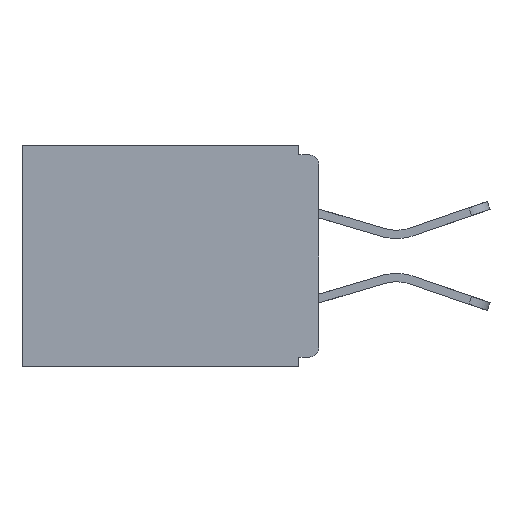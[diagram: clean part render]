
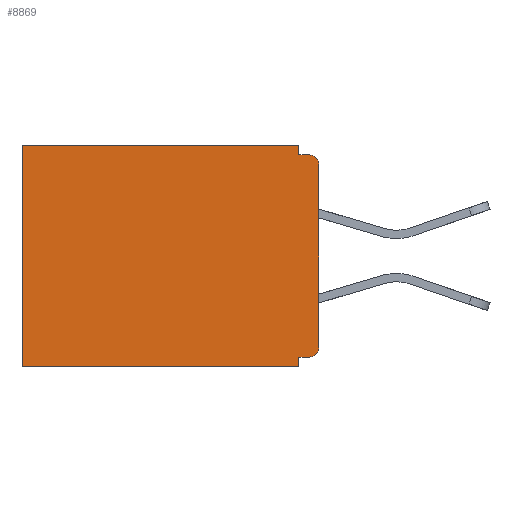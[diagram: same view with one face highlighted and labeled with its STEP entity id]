
A CAD part, left-side view. The second image highlights one B-rep face of the part: STEP entity #8869.
In plain terms, the highlighted planar face has unit normal (-1, 0, 0).
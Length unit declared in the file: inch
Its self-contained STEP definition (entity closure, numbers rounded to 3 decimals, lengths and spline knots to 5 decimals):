
#92 = CIRCLE ( 'NONE', #14591, 0.015 ) ;
#360 = VERTEX_POINT ( 'NONE', #4422 ) ;
#743 = CARTESIAN_POINT ( 'NONE',  ( 0.298, 0.031, -0.343 ) ) ;
#793 = EDGE_CURVE ( 'NONE', #5922, #4514, #23040, .T. ) ;
#941 = ORIENTED_EDGE ( 'NONE', *, *, #23031, .T. ) ;
#2200 = DIRECTION ( 'NONE',  ( -1., 0., 0. ) ) ;
#2765 = DIRECTION ( 'NONE',  ( 0., 0., -1. ) ) ;
#3049 = ORIENTED_EDGE ( 'NONE', *, *, #24527, .F. ) ;
#3358 = EDGE_CURVE ( 'NONE', #14089, #6622, #10035, .T. ) ;
#3411 = CARTESIAN_POINT ( 'NONE',  ( 0.298, 0.46, 0. ) ) ;
#3434 = VECTOR ( 'NONE', #22749, 39.37008 ) ;
#3955 = CARTESIAN_POINT ( 'NONE',  ( 0.298, 0., -0.313 ) ) ;
#4016 = LINE ( 'NONE', #23531, #30515 ) ;
#4174 = DIRECTION ( 'NONE',  ( 1., 0., 0. ) ) ;
#4422 = CARTESIAN_POINT ( 'NONE',  ( 0.298, 0., -0.03 ) ) ;
#4514 = VERTEX_POINT ( 'NONE', #7853 ) ;
#4957 = LINE ( 'NONE', #10898, #3434 ) ;
#5069 = CARTESIAN_POINT ( 'NONE',  ( 0.298, 0.031, -0.343 ) ) ;
#5861 = VECTOR ( 'NONE', #14106, 39.37008 ) ;
#5922 = VERTEX_POINT ( 'NONE', #30896 ) ;
#6333 = ORIENTED_EDGE ( 'NONE', *, *, #13022, .T. ) ;
#6356 = DIRECTION ( 'NONE',  ( -1., 0., 0. ) ) ;
#6622 = VERTEX_POINT ( 'NONE', #3955 ) ;
#7427 = AXIS2_PLACEMENT_3D ( 'NONE', #21047, #4174, #18617 ) ;
#7533 = AXIS2_PLACEMENT_3D ( 'NONE', #28672, #2200, #31295 ) ;
#7853 = CARTESIAN_POINT ( 'NONE',  ( 0.298, 0.015, -0.015 ) ) ;
#7964 = VERTEX_POINT ( 'NONE', #17951 ) ;
#8869 = ADVANCED_FACE ( 'NONE', ( #13870 ), #11394, .F. ) ;
#8871 = ORIENTED_EDGE ( 'NONE', *, *, #20277, .F. ) ;
#10035 = CIRCLE ( 'NONE', #7533, 0.015 ) ;
#10355 = VERTEX_POINT ( 'NONE', #5069 ) ;
#10571 = LINE ( 'NONE', #17393, #11701 ) ;
#10898 = CARTESIAN_POINT ( 'NONE',  ( 0.298, 0., 0. ) ) ;
#11087 = CARTESIAN_POINT ( 'NONE',  ( 0.298, 0., 0. ) ) ;
#11394 = PLANE ( 'NONE',  #7427 ) ;
#11514 = ORIENTED_EDGE ( 'NONE', *, *, #22446, .F. ) ;
#11548 = CARTESIAN_POINT ( 'NONE',  ( 0.298, 0.015, -0.328 ) ) ;
#11701 = VECTOR ( 'NONE', #15026, 39.37008 ) ;
#12139 = VERTEX_POINT ( 'NONE', #27029 ) ;
#12432 = CARTESIAN_POINT ( 'NONE',  ( 0.298, 0.46, 0. ) ) ;
#12556 = EDGE_CURVE ( 'NONE', #30121, #12139, #12691, .T. ) ;
#12691 = LINE ( 'NONE', #12432, #15337 ) ;
#13022 = EDGE_CURVE ( 'NONE', #360, #4514, #92, .T. ) ;
#13870 = FACE_OUTER_BOUND ( 'NONE', #28330, .T. ) ;
#14089 = VERTEX_POINT ( 'NONE', #11548 ) ;
#14106 = DIRECTION ( 'NONE',  ( 0., 0., -1. ) ) ;
#14257 = ORIENTED_EDGE ( 'NONE', *, *, #3358, .T. ) ;
#14581 = ORIENTED_EDGE ( 'NONE', *, *, #793, .F. ) ;
#14591 = AXIS2_PLACEMENT_3D ( 'NONE', #18575, #6356, #28054 ) ;
#15026 = DIRECTION ( 'NONE',  ( 0., 1., 0. ) ) ;
#15048 = DIRECTION ( 'NONE',  ( 0., -1., 0. ) ) ;
#15337 = VECTOR ( 'NONE', #2765, 39.37008 ) ;
#15776 = ORIENTED_EDGE ( 'NONE', *, *, #12556, .T. ) ;
#15803 = ORIENTED_EDGE ( 'NONE', *, *, #16716, .F. ) ;
#16130 = LINE ( 'NONE', #11087, #5861 ) ;
#16716 = EDGE_CURVE ( 'NONE', #14089, #24022, #10571, .T. ) ;
#17195 = CARTESIAN_POINT ( 'NONE',  ( 0.298, 0.031, -0.343 ) ) ;
#17393 = CARTESIAN_POINT ( 'NONE',  ( 0.298, 0., -0.328 ) ) ;
#17511 = CARTESIAN_POINT ( 'NONE',  ( 0.298, 0., -0.015 ) ) ;
#17951 = CARTESIAN_POINT ( 'NONE',  ( 0.298, 0.031, 0. ) ) ;
#18575 = CARTESIAN_POINT ( 'NONE',  ( 0.298, 0.015, -0.03 ) ) ;
#18582 = CARTESIAN_POINT ( 'NONE',  ( 0.298, 0.031, -0.328 ) ) ;
#18617 = DIRECTION ( 'NONE',  ( 0., 0., -1. ) ) ;
#19418 = EDGE_CURVE ( 'NONE', #10355, #12139, #4016, .T. ) ;
#20170 = LINE ( 'NONE', #17195, #25081 ) ;
#20179 = DIRECTION ( 'NONE',  ( 0., 0., -1. ) ) ;
#20277 = EDGE_CURVE ( 'NONE', #360, #6622, #16130, .T. ) ;
#21047 = CARTESIAN_POINT ( 'NONE',  ( 0.298, 0., 0. ) ) ;
#22446 = EDGE_CURVE ( 'NONE', #24022, #10355, #20170, .T. ) ;
#22749 = DIRECTION ( 'NONE',  ( 0., 1., 0. ) ) ;
#23031 = EDGE_CURVE ( 'NONE', #7964, #30121, #4957, .T. ) ;
#23040 = LINE ( 'NONE', #17511, #28676 ) ;
#23531 = CARTESIAN_POINT ( 'NONE',  ( 0.298, 0., -0.343 ) ) ;
#24022 = VERTEX_POINT ( 'NONE', #18582 ) ;
#24527 = EDGE_CURVE ( 'NONE', #7964, #5922, #26461, .T. ) ;
#24593 = DIRECTION ( 'NONE',  ( 0., 0., -1. ) ) ;
#24912 = ORIENTED_EDGE ( 'NONE', *, *, #19418, .F. ) ;
#25081 = VECTOR ( 'NONE', #24593, 39.37008 ) ;
#25921 = DIRECTION ( 'NONE',  ( 0., 1., 0. ) ) ;
#26461 = LINE ( 'NONE', #743, #29073 ) ;
#27029 = CARTESIAN_POINT ( 'NONE',  ( 0.298, 0.46, -0.343 ) ) ;
#28054 = DIRECTION ( 'NONE',  ( 0., 0., -1. ) ) ;
#28330 = EDGE_LOOP ( 'NONE', ( #6333, #14581, #3049, #941, #15776, #24912, #11514, #15803, #14257, #8871 ) ) ;
#28672 = CARTESIAN_POINT ( 'NONE',  ( 0.298, 0.015, -0.313 ) ) ;
#28676 = VECTOR ( 'NONE', #15048, 39.37008 ) ;
#29073 = VECTOR ( 'NONE', #20179, 39.37008 ) ;
#30121 = VERTEX_POINT ( 'NONE', #3411 ) ;
#30515 = VECTOR ( 'NONE', #25921, 39.37008 ) ;
#30896 = CARTESIAN_POINT ( 'NONE',  ( 0.298, 0.031, -0.015 ) ) ;
#31295 = DIRECTION ( 'NONE',  ( 0., 0., -1. ) ) ;
